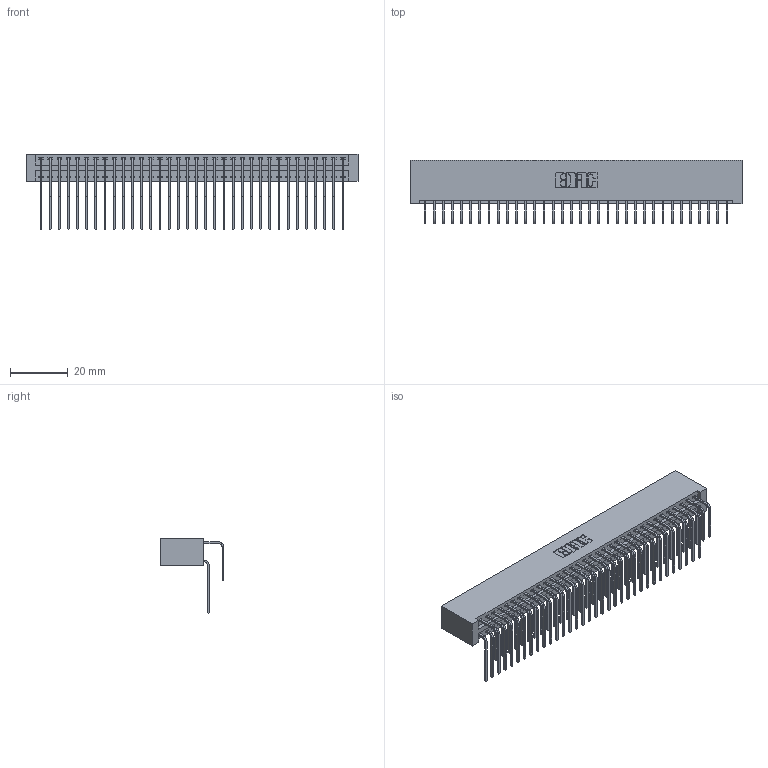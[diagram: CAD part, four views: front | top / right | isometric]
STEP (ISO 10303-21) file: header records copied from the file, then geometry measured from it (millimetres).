
FILE_DESCRIPTION (( 'STEP AP203' ), '1' );
FILE_NAME ('396-068-558-201.STEP', '2019-11-03T10:46:19', ( '' ), ( '' ), 'SwSTEP 2.0', 'SolidWorks 2016', '' );
FILE_SCHEMA (( 'CONFIG_CONTROL_DESIGN' ));
Length unit declared in the file: inch
Products named in the file (4): 396-068-558-201; 346 Part_No Mounting Lugs; 345-292-001_558 Tail - 2; 345-292-001_558 559 Tail - 1
Assembly tree (69 placements, depth 2):
  396-068-558-201
    346 Part_No Mounting Lugs
    345-292-001_558 559 Tail - 1  x34
    345-292-001_558 Tail - 2  x34
Bounding box: 115.19 x 22.16 x 26.16 mm (x, y, z)
Volume: 12135.8 mm3; surface area: 18600.8 mm2
Topology: 69 solids, 69 shells, 3786 faces, 11253 edges, 7410 vertices
Faces by surface type: plane 2588, cylinder 1198
Entity records: 24773 total; most frequent: CARTESIAN_POINT 4143, ORIENTED_EDGE 4026, DIRECTION 3669, EDGE_CURVE 2013, VECTOR 1713, LINE 1713, VERTEX_POINT 1338, AXIS2_PLACEMENT_3D 978
